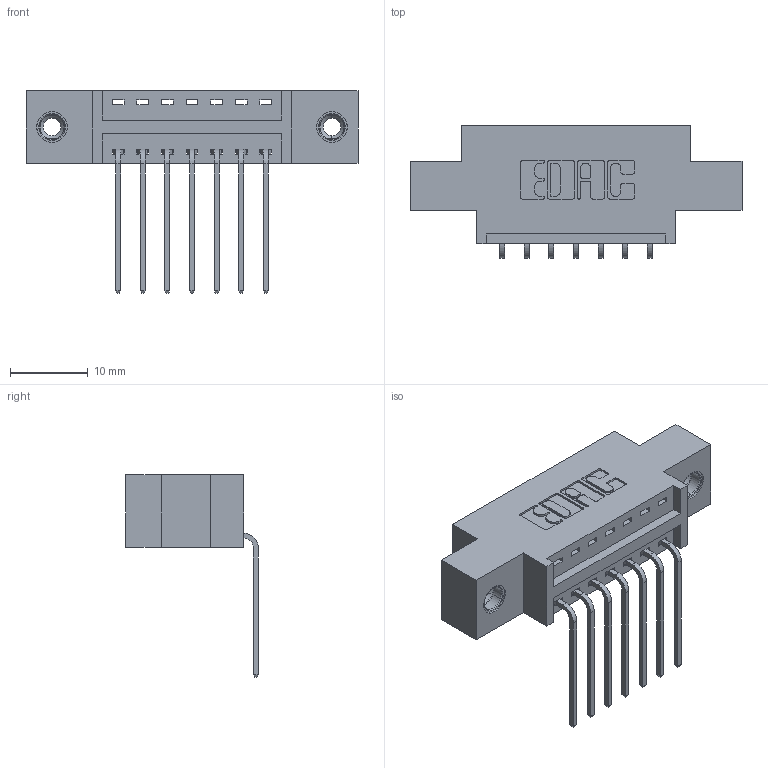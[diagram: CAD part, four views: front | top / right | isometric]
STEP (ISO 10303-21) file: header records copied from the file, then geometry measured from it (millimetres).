
FILE_DESCRIPTION (( 'STEP AP203' ), '1' );
FILE_NAME ('396-007-559-608.STEP', '2019-10-31T19:59:03', ( '' ), ( '' ), 'SwSTEP 2.0', 'SolidWorks 2016', '' );
FILE_SCHEMA (( 'CONFIG_CONTROL_DESIGN' ));
Length unit declared in the file: inch
Products named in the file (4): 346 Part_0.170 Offset - 0.156 Dia-TI; 345-292-001_558 559 Tail - 1; 345-250-001_345-250-003-102; 396-007-559-608
Assembly tree (10 placements, depth 2):
  396-007-559-608
    346 Part_0.170 Offset - 0.156 Dia-TI
    345-292-001_558 559 Tail - 1  x7
    345-250-001_345-250-003-102  x2
Bounding box: 42.8 x 17.08 x 26.16 mm (x, y, z)
Volume: 3717.9 mm3; surface area: 4590.4 mm2
Topology: 10 solids, 10 shells, 606 faces, 1751 edges, 1150 vertices
Faces by surface type: plane 406, cylinder 184, cone 12, torus 4
Entity records: 10458 total; most frequent: CARTESIAN_POINT 1788, ORIENTED_EDGE 1722, DIRECTION 1645, EDGE_CURVE 861, LINE 681, VECTOR 681, VERTEX_POINT 568, AXIS2_PLACEMENT_3D 482
